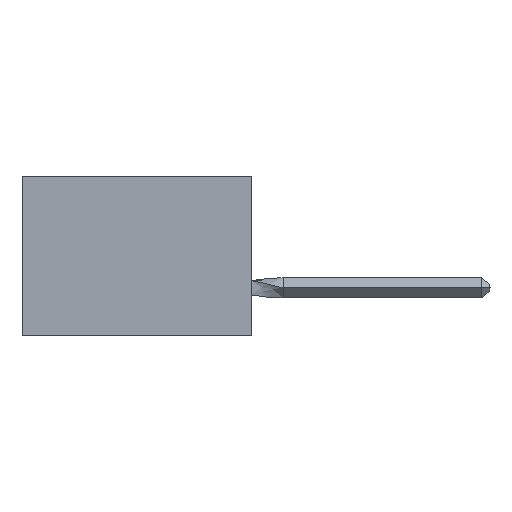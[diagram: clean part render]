
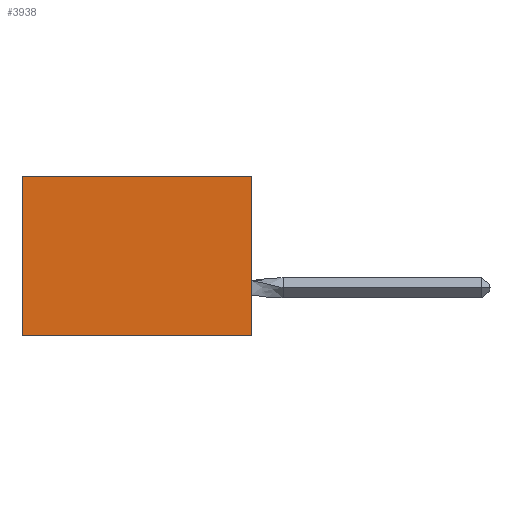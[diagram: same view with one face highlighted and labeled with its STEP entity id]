
A CAD part, left-side view. The second image highlights one B-rep face of the part: STEP entity #3938.
In plain terms, the highlighted planar face has unit normal (-1, 0, 0).
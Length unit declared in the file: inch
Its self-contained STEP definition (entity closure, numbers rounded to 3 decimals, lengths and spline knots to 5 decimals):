
#818 = DIRECTION ( 'NONE',  ( 1., 0., 0. ) ) ;
#948 = CARTESIAN_POINT ( 'NONE',  ( 0.305, 0., -0.5 ) ) ;
#2926 = VERTEX_POINT ( 'NONE', #3738 ) ;
#3056 = VECTOR ( 'NONE', #15097, 39.37008 ) ;
#3490 = EDGE_CURVE ( 'NONE', #10836, #2926, #15218, .T. ) ;
#3516 = LINE ( 'NONE', #11852, #3056 ) ;
#3738 = CARTESIAN_POINT ( 'NONE',  ( 0.305, 0., -0.5 ) ) ;
#3938 = ADVANCED_FACE ( 'NONE', ( #17102 ), #8379, .F. ) ;
#6501 = DIRECTION ( 'NONE',  ( 0., 0., -1. ) ) ;
#6600 = CARTESIAN_POINT ( 'NONE',  ( 0.305, 0.72, 0. ) ) ;
#7575 = VECTOR ( 'NONE', #8534, 39.37008 ) ;
#7663 = DIRECTION ( 'NONE',  ( 0., 1., 0. ) ) ;
#7713 = ORIENTED_EDGE ( 'NONE', *, *, #9998, .T. ) ;
#8379 = PLANE ( 'NONE',  #14013 ) ;
#8534 = DIRECTION ( 'NONE',  ( 0., 0., -1. ) ) ;
#8680 = CARTESIAN_POINT ( 'NONE',  ( 0.305, 0., -0.5 ) ) ;
#9794 = VECTOR ( 'NONE', #6501, 39.37008 ) ;
#9847 = CARTESIAN_POINT ( 'NONE',  ( 0.305, 0., 0. ) ) ;
#9998 = EDGE_CURVE ( 'NONE', #10836, #14362, #3516, .T. ) ;
#10617 = CARTESIAN_POINT ( 'NONE',  ( 0.305, 0., -0.5 ) ) ;
#10762 = LINE ( 'NONE', #10617, #13853 ) ;
#10826 = VERTEX_POINT ( 'NONE', #16110 ) ;
#10836 = VERTEX_POINT ( 'NONE', #9847 ) ;
#11852 = CARTESIAN_POINT ( 'NONE',  ( 0.305, 0., 0. ) ) ;
#12735 = ORIENTED_EDGE ( 'NONE', *, *, #18056, .F. ) ;
#12866 = ORIENTED_EDGE ( 'NONE', *, *, #3490, .F. ) ;
#13733 = EDGE_CURVE ( 'NONE', #14362, #10826, #14324, .T. ) ;
#13853 = VECTOR ( 'NONE', #7663, 39.37008 ) ;
#14013 = AXIS2_PLACEMENT_3D ( 'NONE', #948, #818, #16189 ) ;
#14026 = CARTESIAN_POINT ( 'NONE',  ( 0.305, 0.72, -0.5 ) ) ;
#14324 = LINE ( 'NONE', #14026, #9794 ) ;
#14362 = VERTEX_POINT ( 'NONE', #6600 ) ;
#15097 = DIRECTION ( 'NONE',  ( 0., 1., 0. ) ) ;
#15218 = LINE ( 'NONE', #8680, #7575 ) ;
#16110 = CARTESIAN_POINT ( 'NONE',  ( 0.305, 0.72, -0.5 ) ) ;
#16189 = DIRECTION ( 'NONE',  ( 0., 0., -1. ) ) ;
#17102 = FACE_OUTER_BOUND ( 'NONE', #18149, .T. ) ;
#17986 = ORIENTED_EDGE ( 'NONE', *, *, #13733, .T. ) ;
#18056 = EDGE_CURVE ( 'NONE', #2926, #10826, #10762, .T. ) ;
#18149 = EDGE_LOOP ( 'NONE', ( #17986, #12735, #12866, #7713 ) ) ;
